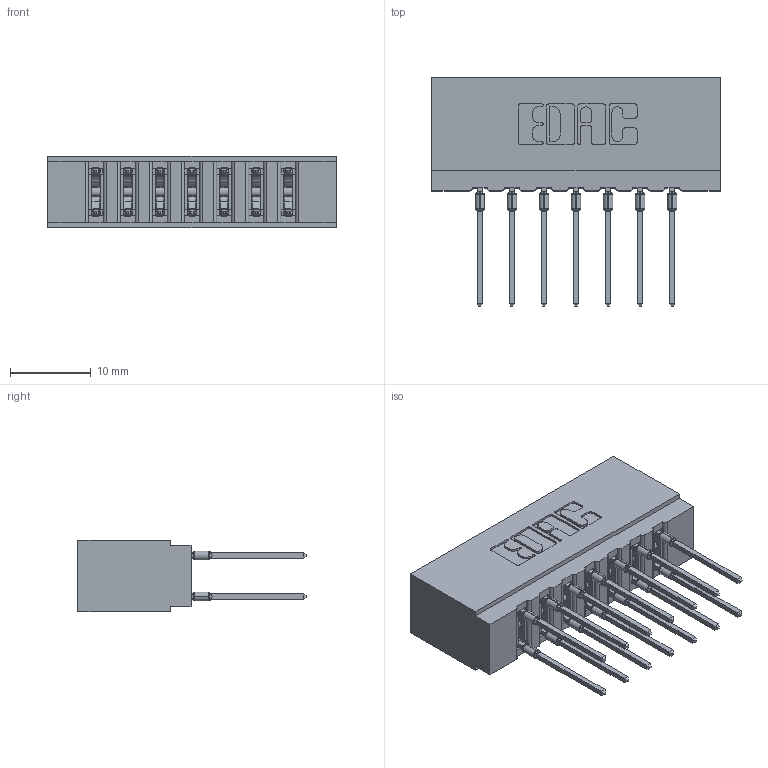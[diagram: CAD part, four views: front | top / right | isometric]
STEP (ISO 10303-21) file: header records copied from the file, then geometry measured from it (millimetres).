
FILE_DESCRIPTION (( 'STEP AP203' ), '1' );
FILE_NAME ('717-014-545-201.STEP', '2026-02-20T17:03:50', ( '' ), ( '' ), 'SwSTEP 2.0', 'SolidWorks 2023', '' );
FILE_SCHEMA (( 'CONFIG_CONTROL_DESIGN' ));
Length unit declared in the file: millimetre
Products named in the file (3): 717-014-545-201; 745-292-001_545; 717 Part_Insulator Option - 06
Assembly tree (15 placements, depth 2):
  717-014-545-201
    717 Part_Insulator Option - 06
    745-292-001_545  x14
Bounding box: 35.61 x 28.18 x 8.89 mm (x, y, z)
Volume: 3279.6 mm3; surface area: 4784.5 mm2
Topology: 15 solids, 15 shells, 1354 faces, 3639 edges, 2294 vertices
Faces by surface type: plane 705, cylinder 285, bspline 280, torus 84
Entity records: 16725 total; most frequent: CARTESIAN_POINT 3415, ORIENTED_EDGE 2780, DIRECTION 2460, EDGE_CURVE 1390, LINE 1166, VECTOR 1166, VERTEX_POINT 890, AXIS2_PLACEMENT_3D 647
